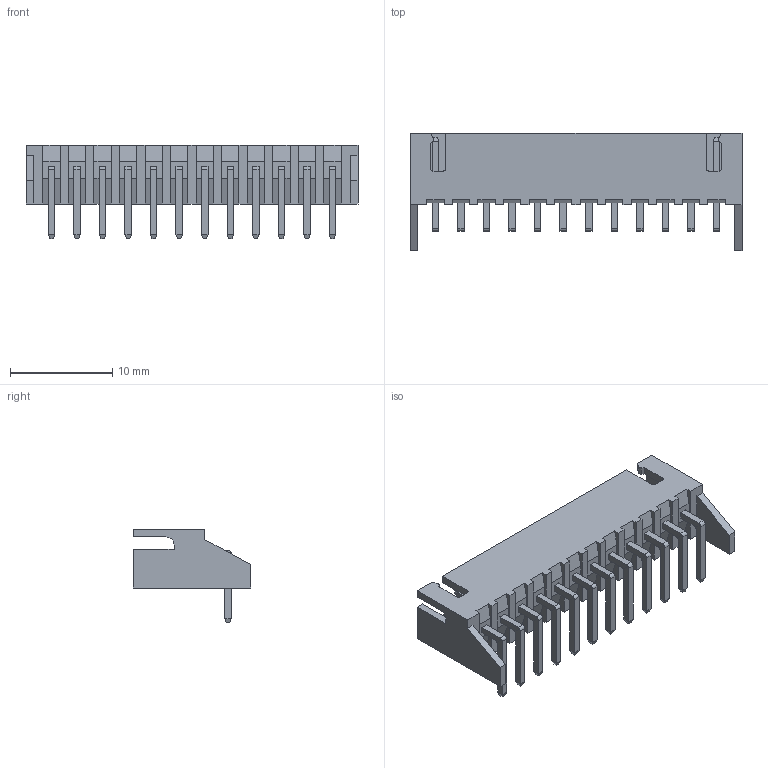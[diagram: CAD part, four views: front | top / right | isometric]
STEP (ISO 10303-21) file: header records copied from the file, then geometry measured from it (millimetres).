
FILE_DESCRIPTION (( 'STEP AP203' ), '1' );
FILE_NAME ('14K-512-416-AD1.STEP', '2024-02-22T15:45:10', ( '' ), ( '' ), 'SwSTEP 2.0', 'SolidWorks 2023', '' );
FILE_SCHEMA (( 'CONFIG_CONTROL_DESIGN' ));
Length unit declared in the file: millimetre
Products named in the file (3): 14K Series Pin with Stabilizer_16; 14K Series Pin Header Insulator with Stabilizer_512; 14K-512-416-AD1
Assembly tree (13 placements, depth 2):
  14K-512-416-AD1
    14K Series Pin Header Insulator with Stabilizer_512
    14K Series Pin with Stabilizer_16  x12
Bounding box: 32.5 x 11.5 x 9.15 mm (x, y, z)
Volume: 653.5 mm3; surface area: 1885.1 mm2
Topology: 13 solids, 13 shells, 430 faces, 1116 edges, 712 vertices
Faces by surface type: plane 397, cylinder 33
Entity records: 6775 total; most frequent: CARTESIAN_POINT 1108, ORIENTED_EDGE 1088, DIRECTION 978, EDGE_CURVE 544, LINE 518, VECTOR 518, VERTEX_POINT 360, AXIS2_PLACEMENT_3D 230
